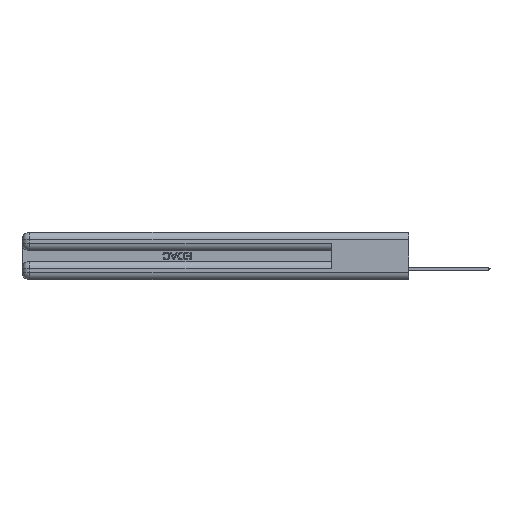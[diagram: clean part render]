
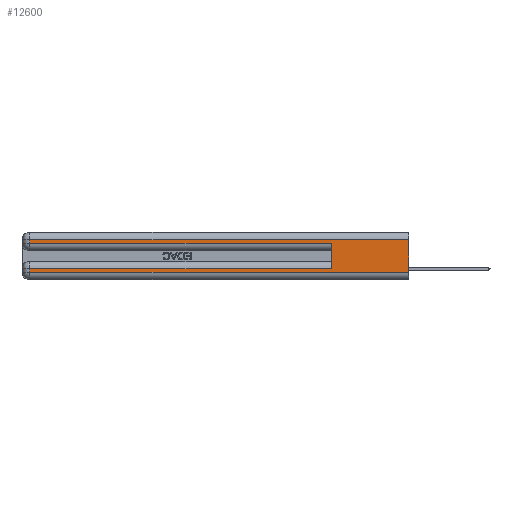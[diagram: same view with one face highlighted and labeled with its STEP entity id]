
A CAD part, left-side view. The second image highlights one B-rep face of the part: STEP entity #12600.
In plain terms, the highlighted planar face has unit normal (-1, 0, 0).
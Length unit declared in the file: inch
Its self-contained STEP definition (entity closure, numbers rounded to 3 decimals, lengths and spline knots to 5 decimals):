
#548 = EDGE_CURVE ( 'NONE', #8998, #26418, #7080, .T. ) ;
#718 = DIRECTION ( 'NONE',  ( 0., 0., -1. ) ) ;
#2139 = DIRECTION ( 'NONE',  ( 0., 0., -1. ) ) ;
#2587 = LINE ( 'NONE', #4475, #8716 ) ;
#3007 = CARTESIAN_POINT ( 'NONE',  ( 0., 2.94, 0.31 ) ) ;
#3035 = VERTEX_POINT ( 'NONE', #26636 ) ;
#4475 = CARTESIAN_POINT ( 'NONE',  ( 0., 0., 0.06 ) ) ;
#4515 = VECTOR ( 'NONE', #25774, 39.37008 ) ;
#6088 = LINE ( 'NONE', #45921, #41693 ) ;
#7080 = LINE ( 'NONE', #11568, #14260 ) ;
#7611 = DIRECTION ( 'NONE',  ( 0., 0., -1. ) ) ;
#8084 = VECTOR ( 'NONE', #34684, 39.37008 ) ;
#8090 = CARTESIAN_POINT ( 'NONE',  ( 0., 0., 0.31 ) ) ;
#8487 = DIRECTION ( 'NONE',  ( 0., 0., 1. ) ) ;
#8716 = VECTOR ( 'NONE', #37302, 39.37008 ) ;
#8998 = VERTEX_POINT ( 'NONE', #42665 ) ;
#9067 = VERTEX_POINT ( 'NONE', #32472 ) ;
#9394 = CARTESIAN_POINT ( 'NONE',  ( 0., 0., 0.085 ) ) ;
#11061 = EDGE_CURVE ( 'NONE', #3035, #28444, #2587, .T. ) ;
#11377 = DIRECTION ( 'NONE',  ( 0., 0., -1. ) ) ;
#11568 = CARTESIAN_POINT ( 'NONE',  ( 0., 0.6, 0.145 ) ) ;
#12600 = ADVANCED_FACE ( 'NONE', ( #45333 ), #33007, .F. ) ;
#13174 = EDGE_CURVE ( 'NONE', #21309, #28444, #42966, .T. ) ;
#13482 = CARTESIAN_POINT ( 'NONE',  ( 0., 2.94, 0.37 ) ) ;
#14260 = VECTOR ( 'NONE', #8487, 39.37008 ) ;
#18411 = ORIENTED_EDGE ( 'NONE', *, *, #24467, .T. ) ;
#19139 = EDGE_CURVE ( 'NONE', #21434, #26418, #32372, .T. ) ;
#20526 = VECTOR ( 'NONE', #2139, 39.37008 ) ;
#21309 = VERTEX_POINT ( 'NONE', #23407 ) ;
#21382 = ORIENTED_EDGE ( 'NONE', *, *, #21704, .T. ) ;
#21434 = VERTEX_POINT ( 'NONE', #28219 ) ;
#21704 = EDGE_CURVE ( 'NONE', #32552, #21434, #30043, .T. ) ;
#22595 = EDGE_CURVE ( 'NONE', #9067, #3035, #6088, .T. ) ;
#22871 = ORIENTED_EDGE ( 'NONE', *, *, #22595, .T. ) ;
#22875 = VECTOR ( 'NONE', #31785, 39.37008 ) ;
#23407 = CARTESIAN_POINT ( 'NONE',  ( 0., 0., 0.31 ) ) ;
#23458 = LINE ( 'NONE', #8090, #4515 ) ;
#24467 = EDGE_CURVE ( 'NONE', #8998, #9067, #27035, .T. ) ;
#25278 = EDGE_LOOP ( 'NONE', ( #38722, #38988, #21382, #34320, #40593, #18411, #22871, #39073 ) ) ;
#25774 = DIRECTION ( 'NONE',  ( 0., 1., 0. ) ) ;
#26418 = VERTEX_POINT ( 'NONE', #39584 ) ;
#26636 = CARTESIAN_POINT ( 'NONE',  ( 0., 2.94, 0.06 ) ) ;
#27035 = LINE ( 'NONE', #9394, #8084 ) ;
#28219 = CARTESIAN_POINT ( 'NONE',  ( 0., 2.94, 0.285 ) ) ;
#28444 = VERTEX_POINT ( 'NONE', #32155 ) ;
#29323 = AXIS2_PLACEMENT_3D ( 'NONE', #43576, #36551, #11377 ) ;
#30043 = LINE ( 'NONE', #13482, #20526 ) ;
#31785 = DIRECTION ( 'NONE',  ( 0., -1., 0. ) ) ;
#32155 = CARTESIAN_POINT ( 'NONE',  ( 0., 0., 0.06 ) ) ;
#32372 = LINE ( 'NONE', #35023, #22875 ) ;
#32472 = CARTESIAN_POINT ( 'NONE',  ( 0., 2.94, 0.085 ) ) ;
#32552 = VERTEX_POINT ( 'NONE', #3007 ) ;
#33007 = PLANE ( 'NONE',  #29323 ) ;
#34120 = EDGE_CURVE ( 'NONE', #21309, #32552, #23458, .T. ) ;
#34320 = ORIENTED_EDGE ( 'NONE', *, *, #19139, .T. ) ;
#34643 = VECTOR ( 'NONE', #718, 39.37008 ) ;
#34684 = DIRECTION ( 'NONE',  ( 0., 1., 0. ) ) ;
#35023 = CARTESIAN_POINT ( 'NONE',  ( 0., 0., 0.285 ) ) ;
#36551 = DIRECTION ( 'NONE',  ( 1., 0., 0. ) ) ;
#37302 = DIRECTION ( 'NONE',  ( 0., -1., 0. ) ) ;
#38722 = ORIENTED_EDGE ( 'NONE', *, *, #13174, .F. ) ;
#38988 = ORIENTED_EDGE ( 'NONE', *, *, #34120, .T. ) ;
#39073 = ORIENTED_EDGE ( 'NONE', *, *, #11061, .T. ) ;
#39373 = CARTESIAN_POINT ( 'NONE',  ( 0., 0., 0.37 ) ) ;
#39584 = CARTESIAN_POINT ( 'NONE',  ( 0., 0.6, 0.285 ) ) ;
#40593 = ORIENTED_EDGE ( 'NONE', *, *, #548, .F. ) ;
#41693 = VECTOR ( 'NONE', #7611, 39.37008 ) ;
#42665 = CARTESIAN_POINT ( 'NONE',  ( 0., 0.6, 0.085 ) ) ;
#42966 = LINE ( 'NONE', #39373, #34643 ) ;
#43576 = CARTESIAN_POINT ( 'NONE',  ( 0., 0., 0.37 ) ) ;
#45333 = FACE_OUTER_BOUND ( 'NONE', #25278, .T. ) ;
#45921 = CARTESIAN_POINT ( 'NONE',  ( 0., 2.94, 0.37 ) ) ;
